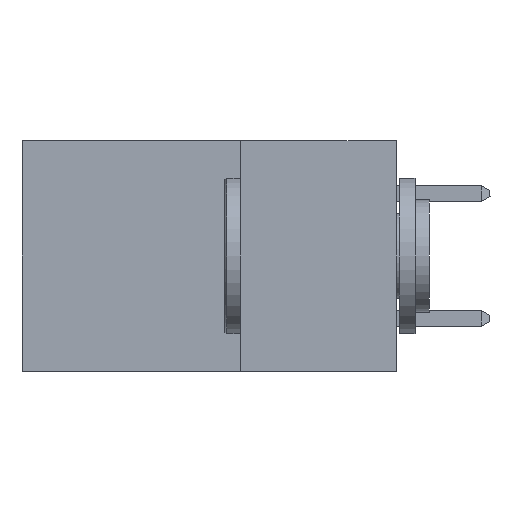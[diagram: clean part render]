
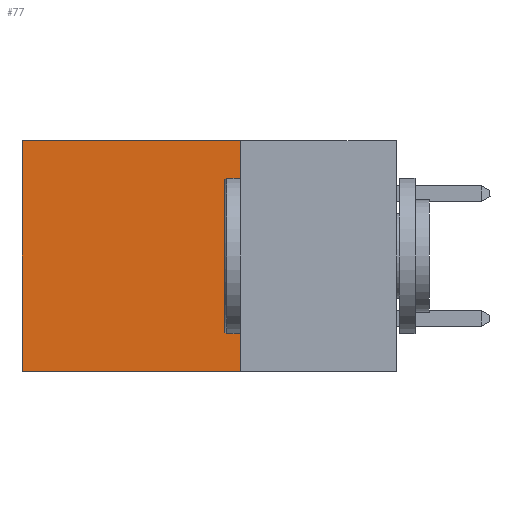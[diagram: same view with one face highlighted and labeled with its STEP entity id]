
A CAD part, left-side view. The second image highlights one B-rep face of the part: STEP entity #77.
In plain terms, the highlighted planar face has unit normal (-1, 0, 0).
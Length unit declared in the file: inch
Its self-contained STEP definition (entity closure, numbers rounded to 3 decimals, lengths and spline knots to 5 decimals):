
#77 = ADVANCED_FACE ( 'NONE', ( #5697 ), #7131, .F. ) ;
#101 = CARTESIAN_POINT ( 'NONE',  ( 0.298, 0.25, 0. ) ) ;
#225 = ORIENTED_EDGE ( 'NONE', *, *, #4664, .F. ) ;
#2359 = LINE ( 'NONE', #4463, #8813 ) ;
#2419 = LINE ( 'NONE', #16919, #19400 ) ;
#3206 = VERTEX_POINT ( 'NONE', #4344 ) ;
#3663 = CARTESIAN_POINT ( 'NONE',  ( 0.298, 0.25, -0.37 ) ) ;
#4344 = CARTESIAN_POINT ( 'NONE',  ( 0.298, 0.6, -0.37 ) ) ;
#4384 = DIRECTION ( 'NONE',  ( 0., 1., 0. ) ) ;
#4463 = CARTESIAN_POINT ( 'NONE',  ( 0.298, 0.25, -0.37 ) ) ;
#4610 = ORIENTED_EDGE ( 'NONE', *, *, #6613, .T. ) ;
#4664 = EDGE_CURVE ( 'NONE', #18581, #5733, #2419, .T. ) ;
#5528 = ORIENTED_EDGE ( 'NONE', *, *, #11258, .F. ) ;
#5697 = FACE_OUTER_BOUND ( 'NONE', #12167, .T. ) ;
#5733 = VERTEX_POINT ( 'NONE', #3663 ) ;
#6123 = EDGE_CURVE ( 'NONE', #18581, #7304, #17880, .T. ) ;
#6613 = EDGE_CURVE ( 'NONE', #7304, #3206, #18666, .T. ) ;
#7131 = PLANE ( 'NONE',  #16897 ) ;
#7217 = CARTESIAN_POINT ( 'NONE',  ( 0.298, 0.25, 0. ) ) ;
#7292 = DIRECTION ( 'NONE',  ( 0., 0., -1. ) ) ;
#7304 = VERTEX_POINT ( 'NONE', #19169 ) ;
#8813 = VECTOR ( 'NONE', #4384, 39.37008 ) ;
#9267 = DIRECTION ( 'NONE',  ( 1., 0., 0. ) ) ;
#9302 = CARTESIAN_POINT ( 'NONE',  ( 0.298, 0.6, 0. ) ) ;
#10176 = CARTESIAN_POINT ( 'NONE',  ( 0.298, 0.25, 0. ) ) ;
#11258 = EDGE_CURVE ( 'NONE', #5733, #3206, #2359, .T. ) ;
#12167 = EDGE_LOOP ( 'NONE', ( #4610, #5528, #225, #12477 ) ) ;
#12477 = ORIENTED_EDGE ( 'NONE', *, *, #6123, .T. ) ;
#14739 = DIRECTION ( 'NONE',  ( 0., 0., -1. ) ) ;
#15256 = VECTOR ( 'NONE', #23263, 39.37008 ) ;
#16897 = AXIS2_PLACEMENT_3D ( 'NONE', #7217, #9267, #7292 ) ;
#16919 = CARTESIAN_POINT ( 'NONE',  ( 0.298, 0.25, 0. ) ) ;
#17880 = LINE ( 'NONE', #10176, #15256 ) ;
#18581 = VERTEX_POINT ( 'NONE', #101 ) ;
#18666 = LINE ( 'NONE', #9302, #19529 ) ;
#19169 = CARTESIAN_POINT ( 'NONE',  ( 0.298, 0.6, 0. ) ) ;
#19400 = VECTOR ( 'NONE', #14739, 39.37008 ) ;
#19529 = VECTOR ( 'NONE', #22383, 39.37008 ) ;
#22383 = DIRECTION ( 'NONE',  ( 0., 0., -1. ) ) ;
#23263 = DIRECTION ( 'NONE',  ( 0., 1., 0. ) ) ;
